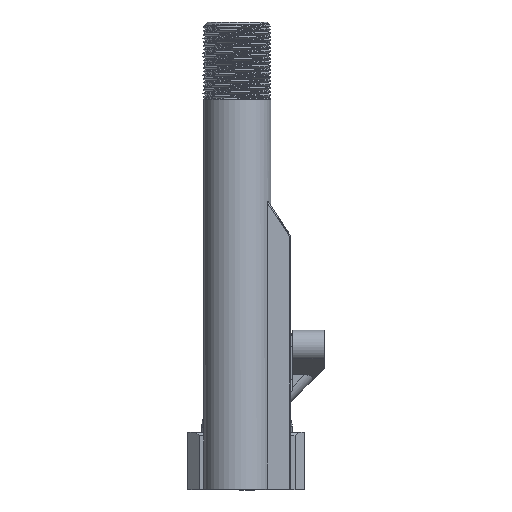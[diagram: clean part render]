
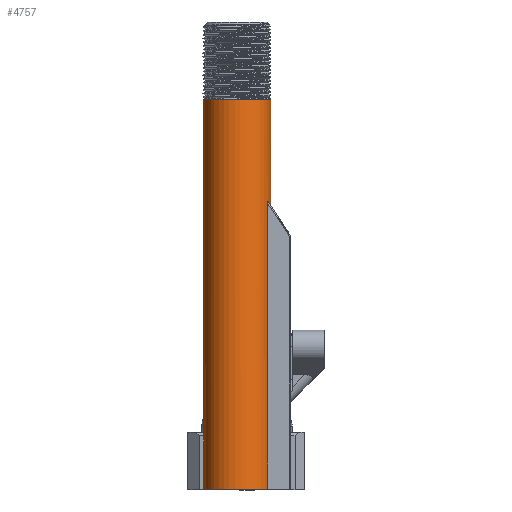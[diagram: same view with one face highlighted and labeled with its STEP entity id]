
A CAD part, left-side view. The second image highlights one B-rep face of the part: STEP entity #4757.
In plain terms, the highlighted cylindrical face has radius 14.5 mm (diameter 29 mm), a full revolution.
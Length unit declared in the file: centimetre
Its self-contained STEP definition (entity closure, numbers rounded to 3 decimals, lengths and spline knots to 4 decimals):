
#130=FACE_BOUND($,#1438,.T.);
#394=LINE($,#15146,#714);
#395=LINE($,#19972,#715);
#714=VECTOR($,#5835,12.3693);
#715=VECTOR($,#5888,12.3693);
#953=CYLINDRICAL_SURFACE($,#5119,1.45);
#995=ELLIPSE($,#5120,2.6293,1.45);
#1142=FACE_OUTER_BOUND($,#1437,.T.);
#1437=EDGE_LOOP($,(#3927,#3928,#3929,#3930,#3931,#3932));
#1438=EDGE_LOOP($,(#3933,#3934));
#1740=B_SPLINE_CURVE_WITH_KNOTS($,3,(#19937,#19938,#19939,#19940,#19941,
#19942,#19943,#19944,#19945,#19946,#19947,#19948,#19949,#19950,#19951,#19952),
 .UNSPECIFIED.,.F.,.F.,(4,2,2,2,2,2,2,4),(0.3605,0.3706,
0.3807,0.389,0.3973,0.4122,
0.4271,0.4569),.UNSPECIFIED.);
#1741=B_SPLINE_CURVE_WITH_KNOTS($,3,(#19956,#19957,#19958,#19959,#19960,
#19961,#19962,#19963,#19964,#19965,#19966,#19967,#19968,#19969,#19970,#19971),
 .UNSPECIFIED.,.F.,.F.,(4,2,2,2,2,2,2,4),(0.,0.0278,
0.0417,0.0556,0.0649,0.0741,
0.085,0.0958),.UNSPECIFIED.);
#1840=CIRCLE($,#5082,1.45);
#1855=CIRCLE($,#5118,1.45);
#1856=CIRCLE($,#5121,1.45);
#2128=VERTEX_POINT($,#15117);
#2129=VERTEX_POINT($,#15119);
#2134=VERTEX_POINT($,#15144);
#2243=VERTEX_POINT($,#19878);
#2244=VERTEX_POINT($,#19897);
#2245=VERTEX_POINT($,#19936);
#2246=VERTEX_POINT($,#19953);
#2247=VERTEX_POINT($,#19955);
#2741=EDGE_CURVE($,#2129,#2128,#1840,.T.);
#2755=EDGE_CURVE($,#2134,#2128,#394,.T.);
#2868=EDGE_CURVE($,#2243,#2244,#1855,.T.);
#2869=EDGE_CURVE($,#2134,#2245,#1740,.F.);
#2870=EDGE_CURVE($,#2246,#2245,#995,.T.);
#2871=EDGE_CURVE($,#2246,#2247,#1741,.F.);
#2872=EDGE_CURVE($,#2129,#2247,#395,.T.);
#2873=EDGE_CURVE($,#2244,#2243,#1856,.T.);
#3927=ORIENTED_EDGE($,*,*,#2741,.T.);
#3928=ORIENTED_EDGE($,*,*,#2755,.F.);
#3929=ORIENTED_EDGE($,*,*,#2869,.T.);
#3930=ORIENTED_EDGE($,*,*,#2870,.F.);
#3931=ORIENTED_EDGE($,*,*,#2871,.T.);
#3932=ORIENTED_EDGE($,*,*,#2872,.F.);
#3933=ORIENTED_EDGE($,*,*,#2868,.T.);
#3934=ORIENTED_EDGE($,*,*,#2873,.T.);
#4757=ADVANCED_FACE($,(#1142,#130),#953,.T.);
#5082=AXIS2_PLACEMENT_3D($,#15120,#5801,#5802);
#5118=AXIS2_PLACEMENT_3D($,#19934,#5882,#5883);
#5119=AXIS2_PLACEMENT_3D($,#19935,#5884,#5885);
#5120=AXIS2_PLACEMENT_3D($,#19954,#5886,#5887);
#5121=AXIS2_PLACEMENT_3D($,#19973,#5889,#5890);
#5801=DIRECTION('center_axis',(0.,0.,1.));
#5802=DIRECTION('ref_axis',(-1.,0.,0.));
#5835=DIRECTION($,(0.,0.,-1.));
#5882=DIRECTION('center_axis',(0.,0.,-1.));
#5883=DIRECTION('ref_axis',(-1.,0.,0.));
#5884=DIRECTION('center_axis',(0.,0.,1.));
#5885=DIRECTION('ref_axis',(-1.,0.,0.));
#5886=DIRECTION('center_axis',(0.,0.834,
-0.551));
#5887=DIRECTION('ref_axis',(0.,-0.551,-0.834));
#5888=DIRECTION($,(0.,0.,1.));
#5889=DIRECTION('center_axis',(0.,0.,-1.));
#5890=DIRECTION('ref_axis',(-1.,0.,0.));
#15117=CARTESIAN_POINT('',(-13.125,-1.3893,2.04));
#15119=CARTESIAN_POINT('',(-11.875,-1.3893,2.04));
#15120=CARTESIAN_POINT('Origin',(-12.5,-0.0809,2.04));
#15144=CARTESIAN_POINT('',(-13.125,-1.3893,14.4093));
#15146=CARTESIAN_POINT($,(-13.125,-1.3893,15.));
#19878=CARTESIAN_POINT('',(-13.7063,0.7238,18.9));
#19897=CARTESIAN_POINT('',(-12.9557,-1.4574,18.9));
#19934=CARTESIAN_POINT('Origin',(-12.5,-0.0809,18.9));
#19935=CARTESIAN_POINT('Origin',(-12.5,-0.0809,15.));
#19936=CARTESIAN_POINT('',(-13.075,-1.412,14.4656));
#19937=CARTESIAN_POINT('Ctrl Pts',(-13.075,-1.412,14.4656));
#19938=CARTESIAN_POINT('Ctrl Pts',(-13.0776,-1.4108,
14.4673));
#19939=CARTESIAN_POINT('Ctrl Pts',(-13.0807,-1.4095,14.469));
#19940=CARTESIAN_POINT('Ctrl Pts',(-13.087,-1.4067,
14.4711));
#19941=CARTESIAN_POINT('Ctrl Pts',(-13.0903,-1.4053,
14.4716));
#19942=CARTESIAN_POINT('Ctrl Pts',(-13.0959,-1.4027,
14.4714));
#19943=CARTESIAN_POINT('Ctrl Pts',(-13.0986,-1.4015,
14.4708));
#19944=CARTESIAN_POINT('Ctrl Pts',(-13.1037,-1.3992,
14.4687));
#19945=CARTESIAN_POINT('Ctrl Pts',(-13.106,-1.3981,
14.4671));
#19946=CARTESIAN_POINT('Ctrl Pts',(-13.1115,-1.3956,14.4622));
#19947=CARTESIAN_POINT('Ctrl Pts',(-13.1142,-1.3944,
14.4584));
#19948=CARTESIAN_POINT('Ctrl Pts',(-13.1186,-1.3923,14.4497));
#19949=CARTESIAN_POINT('Ctrl Pts',(-13.1202,-1.3915,
14.445));
#19950=CARTESIAN_POINT('Ctrl Pts',(-13.1241,-1.3897,
14.4301));
#19951=CARTESIAN_POINT('Ctrl Pts',(-13.125,-1.3893,14.4193));
#19952=CARTESIAN_POINT('Ctrl Pts',(-13.125,-1.3893,14.4093));
#19953=CARTESIAN_POINT('',(-11.925,-1.412,14.4656));
#19954=CARTESIAN_POINT('Origin',(-12.5,-0.0809,16.4792));
#19955=CARTESIAN_POINT('',(-11.875,-1.3893,14.4093));
#19956=CARTESIAN_POINT('Ctrl Pts',(-11.875,-1.3893,14.4093));
#19957=CARTESIAN_POINT('Ctrl Pts',(-11.875,-1.3893,14.4186));
#19958=CARTESIAN_POINT('Ctrl Pts',(-11.8758,-1.3896,
14.4287));
#19959=CARTESIAN_POINT('Ctrl Pts',(-11.8791,-1.3912,14.4429));
#19960=CARTESIAN_POINT('Ctrl Pts',(-11.8806,-1.3919,14.4474));
#19961=CARTESIAN_POINT('Ctrl Pts',(-11.8844,-1.3937,
14.4559));
#19962=CARTESIAN_POINT('Ctrl Pts',(-11.8867,-1.3948,
14.4597));
#19963=CARTESIAN_POINT('Ctrl Pts',(-11.8916,-1.3971,
14.4652));
#19964=CARTESIAN_POINT('Ctrl Pts',(-11.8941,-1.3982,
14.4673));
#19965=CARTESIAN_POINT('Ctrl Pts',(-11.8994,-1.4007,
14.4702));
#19966=CARTESIAN_POINT('Ctrl Pts',(-11.9024,-1.402,
14.4711));
#19967=CARTESIAN_POINT('Ctrl Pts',(-11.9085,-1.4047,
14.4717));
#19968=CARTESIAN_POINT('Ctrl Pts',(-11.912,-1.4063,
14.4713));
#19969=CARTESIAN_POINT('Ctrl Pts',(-11.9189,-1.4093,
14.4692));
#19970=CARTESIAN_POINT('Ctrl Pts',(-11.9222,-1.4108,14.4675));
#19971=CARTESIAN_POINT('Ctrl Pts',(-11.925,-1.412,14.4656));
#19972=CARTESIAN_POINT($,(-11.875,-1.3893,15.));
#19973=CARTESIAN_POINT('Origin',(-12.5,-0.0809,18.9));
